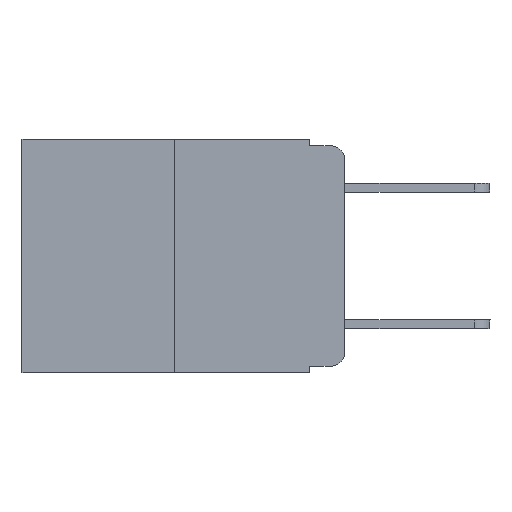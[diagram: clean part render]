
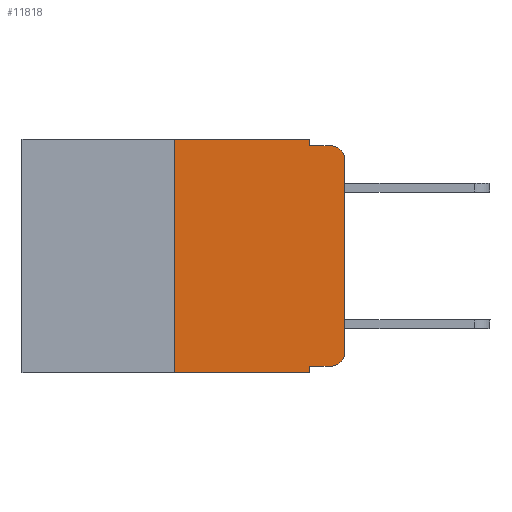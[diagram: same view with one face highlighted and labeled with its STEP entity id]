
A CAD part, left-side view. The second image highlights one B-rep face of the part: STEP entity #11818.
In plain terms, the highlighted planar face has unit normal (-1, 0, 0).
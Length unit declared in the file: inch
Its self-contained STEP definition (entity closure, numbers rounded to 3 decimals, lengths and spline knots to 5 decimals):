
#314 = AXIS2_PLACEMENT_3D ( 'NONE', #18600, #11175, #16870 ) ;
#376 = VECTOR ( 'NONE', #11866, 39.37008 ) ;
#488 = CARTESIAN_POINT ( 'NONE',  ( 0., 0.051, -0.333 ) ) ;
#709 = CARTESIAN_POINT ( 'NONE',  ( 0., 0.051, -0.01 ) ) ;
#754 = DIRECTION ( 'NONE',  ( 0., 0., -1. ) ) ;
#1073 = VECTOR ( 'NONE', #12307, 39.37008 ) ;
#1110 = CARTESIAN_POINT ( 'NONE',  ( 0., 0.473, -0.343 ) ) ;
#1268 = CARTESIAN_POINT ( 'NONE',  ( 0., 0.25, 0. ) ) ;
#1500 = ORIENTED_EDGE ( 'NONE', *, *, #15878, .T. ) ;
#1635 = EDGE_CURVE ( 'NONE', #16964, #16577, #13251, .T. ) ;
#1786 = CIRCLE ( 'NONE', #314, 0.02 ) ;
#1791 = CARTESIAN_POINT ( 'NONE',  ( 0., 0.473, 0. ) ) ;
#2396 = VECTOR ( 'NONE', #4643, 39.37008 ) ;
#2426 = EDGE_CURVE ( 'NONE', #14937, #17925, #8263, .T. ) ;
#3202 = CIRCLE ( 'NONE', #7858, 0.02 ) ;
#3325 = CARTESIAN_POINT ( 'NONE',  ( 0., 0.051, 0. ) ) ;
#3384 = CARTESIAN_POINT ( 'NONE',  ( 0., 0.02, -0.03 ) ) ;
#3462 = LINE ( 'NONE', #1791, #11541 ) ;
#3870 = EDGE_CURVE ( 'NONE', #16738, #9121, #17880, .T. ) ;
#4424 = EDGE_CURVE ( 'NONE', #11642, #18568, #12678, .T. ) ;
#4643 = DIRECTION ( 'NONE',  ( 0., -1., 0. ) ) ;
#4683 = DIRECTION ( 'NONE',  ( 0., -1., 0. ) ) ;
#4734 = CARTESIAN_POINT ( 'NONE',  ( 0., 0.051, 0. ) ) ;
#4793 = DIRECTION ( 'NONE',  ( 0., 0., -1. ) ) ;
#5317 = ORIENTED_EDGE ( 'NONE', *, *, #9776, .T. ) ;
#5399 = CARTESIAN_POINT ( 'NONE',  ( 0., 0.051, -0.01 ) ) ;
#5580 = CARTESIAN_POINT ( 'NONE',  ( 0., 0.051, -0.333 ) ) ;
#6002 = DIRECTION ( 'NONE',  ( 0., 0., 1. ) ) ;
#6084 = DIRECTION ( 'NONE',  ( 0., 0., 1. ) ) ;
#6217 = CARTESIAN_POINT ( 'NONE',  ( 0., 0., -0.313 ) ) ;
#6525 = VERTEX_POINT ( 'NONE', #9376 ) ;
#7163 = CARTESIAN_POINT ( 'NONE',  ( 0., 0.02, -0.333 ) ) ;
#7249 = ORIENTED_EDGE ( 'NONE', *, *, #3870, .F. ) ;
#7833 = VECTOR ( 'NONE', #16975, 39.37008 ) ;
#7853 = EDGE_CURVE ( 'NONE', #16738, #12170, #17893, .T. ) ;
#7858 = AXIS2_PLACEMENT_3D ( 'NONE', #3384, #13421, #4793 ) ;
#7920 = ORIENTED_EDGE ( 'NONE', *, *, #1635, .F. ) ;
#8213 = CARTESIAN_POINT ( 'NONE',  ( 0., 0.051, 0. ) ) ;
#8263 = LINE ( 'NONE', #8213, #7833 ) ;
#9120 = CARTESIAN_POINT ( 'NONE',  ( 0., 0.473, 0. ) ) ;
#9121 = VERTEX_POINT ( 'NONE', #12119 ) ;
#9169 = ORIENTED_EDGE ( 'NONE', *, *, #2426, .F. ) ;
#9305 = CARTESIAN_POINT ( 'NONE',  ( 0., 0., -0.03 ) ) ;
#9376 = CARTESIAN_POINT ( 'NONE',  ( 0., 0.02, -0.01 ) ) ;
#9435 = AXIS2_PLACEMENT_3D ( 'NONE', #9120, #16423, #754 ) ;
#9440 = VECTOR ( 'NONE', #6084, 39.37008 ) ;
#9776 = EDGE_CURVE ( 'NONE', #18568, #6525, #3202, .T. ) ;
#11109 = DIRECTION ( 'NONE',  ( 0., -1., 0. ) ) ;
#11175 = DIRECTION ( 'NONE',  ( -1., 0., 0. ) ) ;
#11512 = ORIENTED_EDGE ( 'NONE', *, *, #16200, .F. ) ;
#11541 = VECTOR ( 'NONE', #4683, 39.37008 ) ;
#11642 = VERTEX_POINT ( 'NONE', #6217 ) ;
#11818 = ADVANCED_FACE ( 'NONE', ( #15230 ), #18115, .F. ) ;
#11866 = DIRECTION ( 'NONE',  ( 0., 0., -1. ) ) ;
#12119 = CARTESIAN_POINT ( 'NONE',  ( 0., 0.051, -0.343 ) ) ;
#12170 = VERTEX_POINT ( 'NONE', #7163 ) ;
#12307 = DIRECTION ( 'NONE',  ( 0., -1., 0. ) ) ;
#12678 = LINE ( 'NONE', #16123, #13338 ) ;
#12684 = VECTOR ( 'NONE', #11109, 39.37008 ) ;
#13138 = LINE ( 'NONE', #1110, #12684 ) ;
#13164 = LINE ( 'NONE', #709, #1073 ) ;
#13227 = EDGE_LOOP ( 'NONE', ( #16645, #5317, #14467, #9169, #11512, #7920, #1500, #7249, #15153, #14626 ) ) ;
#13251 = LINE ( 'NONE', #1268, #9440 ) ;
#13338 = VECTOR ( 'NONE', #6002, 39.37008 ) ;
#13382 = EDGE_CURVE ( 'NONE', #12170, #11642, #1786, .T. ) ;
#13421 = DIRECTION ( 'NONE',  ( -1., 0., 0. ) ) ;
#14405 = EDGE_CURVE ( 'NONE', #17925, #6525, #13164, .T. ) ;
#14467 = ORIENTED_EDGE ( 'NONE', *, *, #14405, .F. ) ;
#14626 = ORIENTED_EDGE ( 'NONE', *, *, #13382, .T. ) ;
#14644 = CARTESIAN_POINT ( 'NONE',  ( 0., 0.25, -0.343 ) ) ;
#14937 = VERTEX_POINT ( 'NONE', #3325 ) ;
#15153 = ORIENTED_EDGE ( 'NONE', *, *, #7853, .T. ) ;
#15230 = FACE_OUTER_BOUND ( 'NONE', #13227, .T. ) ;
#15878 = EDGE_CURVE ( 'NONE', #16964, #9121, #13138, .T. ) ;
#16123 = CARTESIAN_POINT ( 'NONE',  ( 0., 0., 0. ) ) ;
#16200 = EDGE_CURVE ( 'NONE', #16577, #14937, #3462, .T. ) ;
#16423 = DIRECTION ( 'NONE',  ( 1., 0., 0. ) ) ;
#16577 = VERTEX_POINT ( 'NONE', #16734 ) ;
#16645 = ORIENTED_EDGE ( 'NONE', *, *, #4424, .T. ) ;
#16734 = CARTESIAN_POINT ( 'NONE',  ( 0., 0.25, 0. ) ) ;
#16738 = VERTEX_POINT ( 'NONE', #5580 ) ;
#16870 = DIRECTION ( 'NONE',  ( 0., 0., -1. ) ) ;
#16964 = VERTEX_POINT ( 'NONE', #14644 ) ;
#16975 = DIRECTION ( 'NONE',  ( 0., 0., -1. ) ) ;
#17880 = LINE ( 'NONE', #4734, #376 ) ;
#17893 = LINE ( 'NONE', #488, #2396 ) ;
#17925 = VERTEX_POINT ( 'NONE', #5399 ) ;
#18115 = PLANE ( 'NONE',  #9435 ) ;
#18568 = VERTEX_POINT ( 'NONE', #9305 ) ;
#18600 = CARTESIAN_POINT ( 'NONE',  ( 0., 0.02, -0.313 ) ) ;
